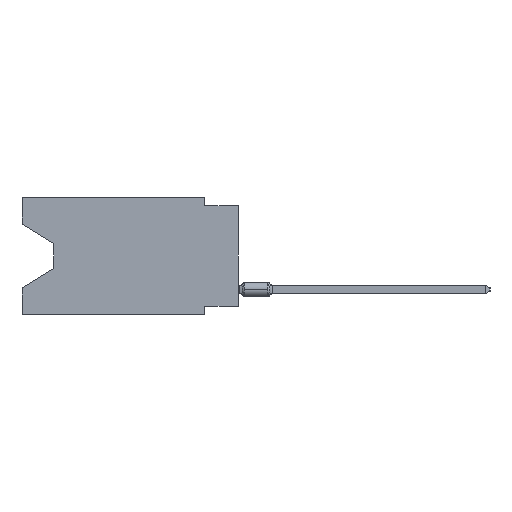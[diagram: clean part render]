
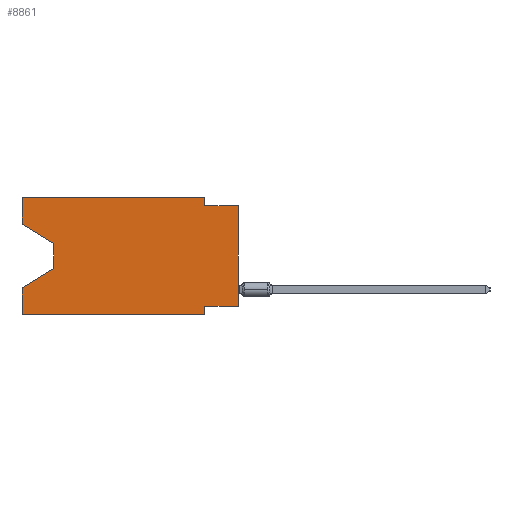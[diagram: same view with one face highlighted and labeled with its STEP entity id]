
A CAD part, left-side view. The second image highlights one B-rep face of the part: STEP entity #8861.
In plain terms, the highlighted planar face has unit normal (-1, 0, 0).
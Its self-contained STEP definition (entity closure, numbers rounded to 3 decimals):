
#943 = CARTESIAN_POINT ( 'NONE',  ( 0., 2.54, 0. ) ) ;
#2533 = VECTOR ( 'NONE', #45413, 1000. ) ;
#3800 = EDGE_CURVE ( 'NONE', #98483, #29813, #79670, .T. ) ;
#5347 = DIRECTION ( 'NONE',  ( 0., -1., 0. ) ) ;
#7753 = VERTEX_POINT ( 'NONE', #60078 ) ;
#8861 = ADVANCED_FACE ( 'NONE', ( #82765 ), #39252, .F. ) ;
#9007 = DIRECTION ( 'NONE',  ( 0., 0., 1. ) ) ;
#9098 = VECTOR ( 'NONE', #25770, 1000. ) ;
#9118 = ORIENTED_EDGE ( 'NONE', *, *, #26881, .T. ) ;
#9925 = CARTESIAN_POINT ( 'NONE',  ( 0., 13.97, -5.385 ) ) ;
#11164 = LINE ( 'NONE', #11687, #111289 ) ;
#11687 = CARTESIAN_POINT ( 'NONE',  ( 0., 0., -8.255 ) ) ;
#12855 = LINE ( 'NONE', #45658, #69567 ) ;
#12893 = LINE ( 'NONE', #47356, #78910 ) ;
#13682 = ORIENTED_EDGE ( 'NONE', *, *, #28776, .T. ) ;
#13796 = EDGE_CURVE ( 'NONE', #56488, #26976, #88623, .T. ) ;
#14050 = CARTESIAN_POINT ( 'NONE',  ( 0., 2.54, -8.89 ) ) ;
#16070 = CARTESIAN_POINT ( 'NONE',  ( 0., 16.383, 0. ) ) ;
#16246 = CARTESIAN_POINT ( 'NONE',  ( 0., 0., -0.635 ) ) ;
#18430 = CARTESIAN_POINT ( 'NONE',  ( 0., 16.383, -6.852 ) ) ;
#21191 = ORIENTED_EDGE ( 'NONE', *, *, #48882, .T. ) ;
#22315 = ORIENTED_EDGE ( 'NONE', *, *, #63142, .F. ) ;
#23852 = CARTESIAN_POINT ( 'NONE',  ( 0., 2.54, 0. ) ) ;
#24721 = LINE ( 'NONE', #943, #38445 ) ;
#25032 = EDGE_LOOP ( 'NONE', ( #21191, #45409, #13682, #22315, #9118, #56665, #47594, #98401, #85190, #65354, #68100, #74530 ) ) ;
#25449 = VERTEX_POINT ( 'NONE', #83402 ) ;
#25770 = DIRECTION ( 'NONE',  ( 0., -0.855, -0.519 ) ) ;
#26881 = EDGE_CURVE ( 'NONE', #25449, #7753, #100975, .T. ) ;
#26976 = VERTEX_POINT ( 'NONE', #9925 ) ;
#28605 = VECTOR ( 'NONE', #9007, 1000. ) ;
#28776 = EDGE_CURVE ( 'NONE', #26976, #107098, #53891, .T. ) ;
#29813 = VERTEX_POINT ( 'NONE', #16246 ) ;
#31874 = DIRECTION ( 'NONE',  ( 0., 0., -1. ) ) ;
#32924 = CARTESIAN_POINT ( 'NONE',  ( 0., 16.383, 0. ) ) ;
#33140 = CARTESIAN_POINT ( 'NONE',  ( 0., 16.383, -2.038 ) ) ;
#33877 = VECTOR ( 'NONE', #67084, 1000. ) ;
#33893 = LINE ( 'NONE', #94361, #28605 ) ;
#34077 = CARTESIAN_POINT ( 'NONE',  ( 0., 2.54, -8.255 ) ) ;
#34177 = VERTEX_POINT ( 'NONE', #23852 ) ;
#38445 = VECTOR ( 'NONE', #69933, 1000. ) ;
#39041 = VECTOR ( 'NONE', #65476, 1000. ) ;
#39252 = PLANE ( 'NONE',  #69901 ) ;
#41751 = CARTESIAN_POINT ( 'NONE',  ( 0., 13.97, -3.505 ) ) ;
#43018 = EDGE_CURVE ( 'NONE', #90900, #7753, #82442, .T. ) ;
#45409 = ORIENTED_EDGE ( 'NONE', *, *, #13796, .T. ) ;
#45413 = DIRECTION ( 'NONE',  ( 0., 0.855, -0.519 ) ) ;
#45658 = CARTESIAN_POINT ( 'NONE',  ( 0., 16.383, 0. ) ) ;
#47356 = CARTESIAN_POINT ( 'NONE',  ( 0., 16.383, 0. ) ) ;
#47594 = ORIENTED_EDGE ( 'NONE', *, *, #72141, .F. ) ;
#48288 = CARTESIAN_POINT ( 'NONE',  ( 0., 16.383, 0. ) ) ;
#48882 = EDGE_CURVE ( 'NONE', #86656, #56488, #59698, .T. ) ;
#53604 = EDGE_CURVE ( 'NONE', #34177, #98483, #24721, .T. ) ;
#53891 = LINE ( 'NONE', #88368, #2533 ) ;
#56488 = VERTEX_POINT ( 'NONE', #41751 ) ;
#56665 = ORIENTED_EDGE ( 'NONE', *, *, #43018, .F. ) ;
#58043 = CARTESIAN_POINT ( 'NONE',  ( 0., 16.383, -8.89 ) ) ;
#59698 = LINE ( 'NONE', #33140, #9098 ) ;
#60078 = CARTESIAN_POINT ( 'NONE',  ( 0., 2.54, -8.89 ) ) ;
#61487 = CARTESIAN_POINT ( 'NONE',  ( 0., 0., -8.255 ) ) ;
#62104 = DIRECTION ( 'NONE',  ( 0., -1., 0. ) ) ;
#63142 = EDGE_CURVE ( 'NONE', #25449, #107098, #12893, .T. ) ;
#64444 = EDGE_CURVE ( 'NONE', #68138, #29813, #33893, .T. ) ;
#65354 = ORIENTED_EDGE ( 'NONE', *, *, #53604, .F. ) ;
#65476 = DIRECTION ( 'NONE',  ( 0., 0., -1. ) ) ;
#67084 = DIRECTION ( 'NONE',  ( 0., -1., 0. ) ) ;
#68100 = ORIENTED_EDGE ( 'NONE', *, *, #108209, .F. ) ;
#68138 = VERTEX_POINT ( 'NONE', #61487 ) ;
#69021 = VECTOR ( 'NONE', #62104, 1000. ) ;
#69567 = VECTOR ( 'NONE', #105553, 1000. ) ;
#69901 = AXIS2_PLACEMENT_3D ( 'NONE', #48288, #92360, #31874 ) ;
#69933 = DIRECTION ( 'NONE',  ( 0., 0., -1. ) ) ;
#72141 = EDGE_CURVE ( 'NONE', #68138, #90900, #11164, .T. ) ;
#74530 = ORIENTED_EDGE ( 'NONE', *, *, #98094, .F. ) ;
#75435 = LINE ( 'NONE', #16070, #85276 ) ;
#78910 = VECTOR ( 'NONE', #81840, 1000. ) ;
#79620 = VERTEX_POINT ( 'NONE', #32924 ) ;
#79670 = LINE ( 'NONE', #96048, #69021 ) ;
#81840 = DIRECTION ( 'NONE',  ( 0., 0., 1. ) ) ;
#82442 = LINE ( 'NONE', #14050, #39041 ) ;
#82765 = FACE_OUTER_BOUND ( 'NONE', #25032, .T. ) ;
#83402 = CARTESIAN_POINT ( 'NONE',  ( 0., 16.383, -8.89 ) ) ;
#84876 = DIRECTION ( 'NONE',  ( 0., 0., -1. ) ) ;
#85052 = VECTOR ( 'NONE', #84876, 1000. ) ;
#85190 = ORIENTED_EDGE ( 'NONE', *, *, #3800, .F. ) ;
#85276 = VECTOR ( 'NONE', #5347, 1000. ) ;
#86656 = VERTEX_POINT ( 'NONE', #107239 ) ;
#88368 = CARTESIAN_POINT ( 'NONE',  ( 0., 13.97, -5.385 ) ) ;
#88623 = LINE ( 'NONE', #104463, #85052 ) ;
#90900 = VERTEX_POINT ( 'NONE', #34077 ) ;
#92360 = DIRECTION ( 'NONE',  ( 1., 0., 0. ) ) ;
#94361 = CARTESIAN_POINT ( 'NONE',  ( 0., 0., 0. ) ) ;
#96048 = CARTESIAN_POINT ( 'NONE',  ( 0., 0., -0.635 ) ) ;
#98036 = CARTESIAN_POINT ( 'NONE',  ( 0., 2.54, -0.635 ) ) ;
#98094 = EDGE_CURVE ( 'NONE', #86656, #79620, #12855, .T. ) ;
#98401 = ORIENTED_EDGE ( 'NONE', *, *, #64444, .T. ) ;
#98483 = VERTEX_POINT ( 'NONE', #98036 ) ;
#99262 = DIRECTION ( 'NONE',  ( 0., 1., 0. ) ) ;
#100975 = LINE ( 'NONE', #58043, #33877 ) ;
#104463 = CARTESIAN_POINT ( 'NONE',  ( 0., 13.97, -3.505 ) ) ;
#105553 = DIRECTION ( 'NONE',  ( 0., 0., 1. ) ) ;
#107098 = VERTEX_POINT ( 'NONE', #18430 ) ;
#107239 = CARTESIAN_POINT ( 'NONE',  ( 0., 16.383, -2.038 ) ) ;
#108209 = EDGE_CURVE ( 'NONE', #79620, #34177, #75435, .T. ) ;
#111289 = VECTOR ( 'NONE', #99262, 1000. ) ;
